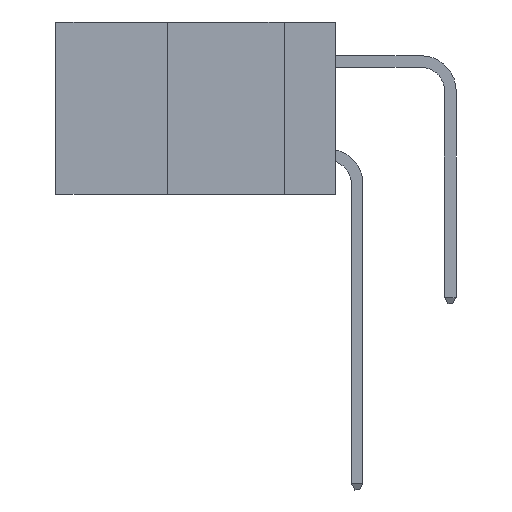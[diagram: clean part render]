
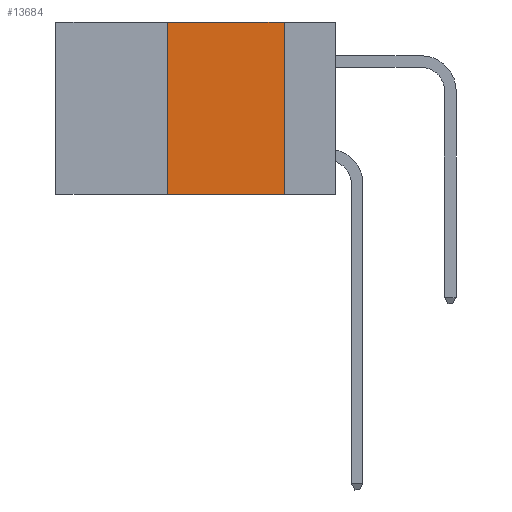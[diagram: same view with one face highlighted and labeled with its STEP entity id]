
A CAD part, left-side view. The second image highlights one B-rep face of the part: STEP entity #13684.
In plain terms, the highlighted planar face has unit normal (-1, 0, 0).
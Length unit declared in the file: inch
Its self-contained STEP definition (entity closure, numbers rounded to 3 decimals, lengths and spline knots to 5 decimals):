
#369 = CARTESIAN_POINT ( 'NONE',  ( 0., 0.36, 0. ) ) ;
#477 = DIRECTION ( 'NONE',  ( 0., 0., 1. ) ) ;
#724 = EDGE_CURVE ( 'NONE', #16953, #2716, #5365, .T. ) ;
#1041 = CARTESIAN_POINT ( 'NONE',  ( 0., 0.6, -0.37 ) ) ;
#1203 = VERTEX_POINT ( 'NONE', #4558 ) ;
#2326 = CARTESIAN_POINT ( 'NONE',  ( 0., 0.11, 0. ) ) ;
#2457 = PLANE ( 'NONE',  #28156 ) ;
#2716 = VERTEX_POINT ( 'NONE', #26644 ) ;
#3823 = VECTOR ( 'NONE', #10653, 39.37008 ) ;
#4462 = CARTESIAN_POINT ( 'NONE',  ( 0., 0.6, 0. ) ) ;
#4558 = CARTESIAN_POINT ( 'NONE',  ( 0., 0.36, 0. ) ) ;
#5018 = LINE ( 'NONE', #2326, #3823 ) ;
#5365 = LINE ( 'NONE', #1041, #22858 ) ;
#7108 = ORIENTED_EDGE ( 'NONE', *, *, #11291, .F. ) ;
#7394 = ORIENTED_EDGE ( 'NONE', *, *, #724, .T. ) ;
#9040 = CARTESIAN_POINT ( 'NONE',  ( 0., 0.36, -0.37 ) ) ;
#10021 = ORIENTED_EDGE ( 'NONE', *, *, #31358, .F. ) ;
#10464 = EDGE_LOOP ( 'NONE', ( #29149, #10021, #7108, #7394 ) ) ;
#10653 = DIRECTION ( 'NONE',  ( 0., 0., -1. ) ) ;
#11291 = EDGE_CURVE ( 'NONE', #16953, #1203, #22743, .T. ) ;
#11819 = DIRECTION ( 'NONE',  ( 0., -1., 0. ) ) ;
#11975 = CARTESIAN_POINT ( 'NONE',  ( 0., 0.6, 0. ) ) ;
#13684 = ADVANCED_FACE ( 'NONE', ( #24873 ), #2457, .F. ) ;
#14169 = DIRECTION ( 'NONE',  ( 0., -1., 0. ) ) ;
#16953 = VERTEX_POINT ( 'NONE', #9040 ) ;
#17386 = LINE ( 'NONE', #4462, #25525 ) ;
#20262 = CARTESIAN_POINT ( 'NONE',  ( 0., 0.11, 0. ) ) ;
#20281 = DIRECTION ( 'NONE',  ( 0., 0., -1. ) ) ;
#21164 = VECTOR ( 'NONE', #477, 39.37008 ) ;
#22743 = LINE ( 'NONE', #369, #21164 ) ;
#22858 = VECTOR ( 'NONE', #14169, 39.37008 ) ;
#24323 = EDGE_CURVE ( 'NONE', #29253, #2716, #5018, .T. ) ;
#24873 = FACE_OUTER_BOUND ( 'NONE', #10464, .T. ) ;
#25525 = VECTOR ( 'NONE', #11819, 39.37008 ) ;
#26644 = CARTESIAN_POINT ( 'NONE',  ( 0., 0.11, -0.37 ) ) ;
#27444 = DIRECTION ( 'NONE',  ( 1., 0., 0. ) ) ;
#28156 = AXIS2_PLACEMENT_3D ( 'NONE', #11975, #27444, #20281 ) ;
#29149 = ORIENTED_EDGE ( 'NONE', *, *, #24323, .F. ) ;
#29253 = VERTEX_POINT ( 'NONE', #20262 ) ;
#31358 = EDGE_CURVE ( 'NONE', #1203, #29253, #17386, .T. ) ;
